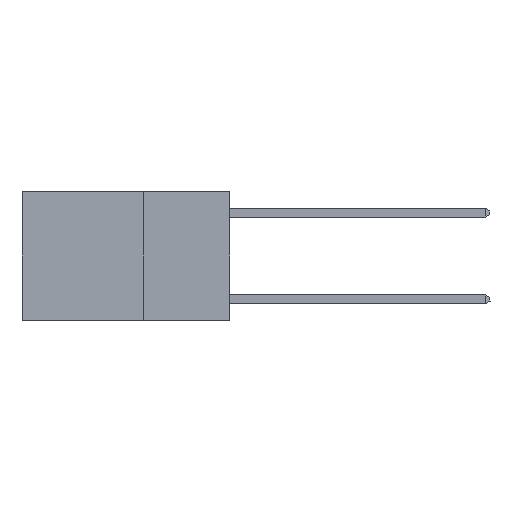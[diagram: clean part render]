
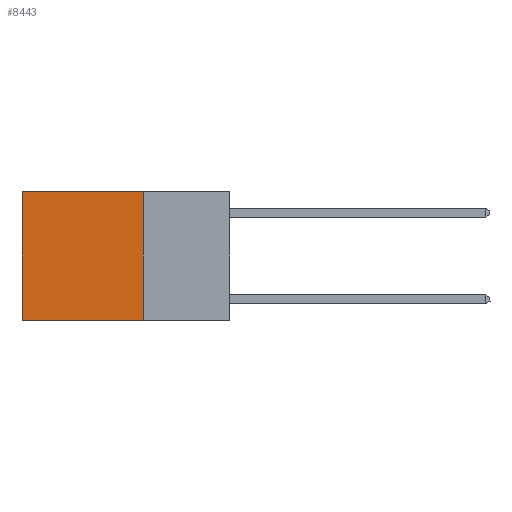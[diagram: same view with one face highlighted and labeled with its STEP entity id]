
A CAD part, left-side view. The second image highlights one B-rep face of the part: STEP entity #8443.
In plain terms, the highlighted planar face has unit normal (-1, 0, 0).
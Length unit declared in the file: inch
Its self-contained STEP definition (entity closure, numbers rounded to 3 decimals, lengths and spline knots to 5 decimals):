
#1500 = DIRECTION ( 'NONE',  ( 0., 1., 0. ) ) ;
#2161 = VECTOR ( 'NONE', #10301, 39.37008 ) ;
#2451 = EDGE_CURVE ( 'NONE', #3620, #8797, #5999, .T. ) ;
#2738 = DIRECTION ( 'NONE',  ( 0., 1., 0. ) ) ;
#3220 = ORIENTED_EDGE ( 'NONE', *, *, #14778, .T. ) ;
#3357 = CARTESIAN_POINT ( 'NONE',  ( 0.2625, 0.25, -0.37 ) ) ;
#3620 = VERTEX_POINT ( 'NONE', #12594 ) ;
#3892 = EDGE_CURVE ( 'NONE', #8797, #12359, #15888, .T. ) ;
#3906 = FACE_OUTER_BOUND ( 'NONE', #12602, .T. ) ;
#4380 = CARTESIAN_POINT ( 'NONE',  ( 0.2625, 0.6, -0.37 ) ) ;
#5059 = ORIENTED_EDGE ( 'NONE', *, *, #3892, .F. ) ;
#5229 = CARTESIAN_POINT ( 'NONE',  ( 0.2625, 0.25, 0. ) ) ;
#5540 = DIRECTION ( 'NONE',  ( 0., 0., -1. ) ) ;
#5999 = LINE ( 'NONE', #5229, #2161 ) ;
#6044 = EDGE_CURVE ( 'NONE', #3620, #12465, #14558, .T. ) ;
#6697 = VECTOR ( 'NONE', #1500, 39.37008 ) ;
#8006 = DIRECTION ( 'NONE',  ( 0., 0., -1. ) ) ;
#8443 = ADVANCED_FACE ( 'NONE', ( #3906 ), #16198, .F. ) ;
#8797 = VERTEX_POINT ( 'NONE', #10371 ) ;
#8907 = LINE ( 'NONE', #12618, #16201 ) ;
#10131 = CARTESIAN_POINT ( 'NONE',  ( 0.2625, 0.25, 0. ) ) ;
#10137 = ORIENTED_EDGE ( 'NONE', *, *, #6044, .T. ) ;
#10271 = CARTESIAN_POINT ( 'NONE',  ( 0.2625, 0.6, 0. ) ) ;
#10301 = DIRECTION ( 'NONE',  ( 0., 0., -1. ) ) ;
#10371 = CARTESIAN_POINT ( 'NONE',  ( 0.2625, 0.25, -0.37 ) ) ;
#11744 = AXIS2_PLACEMENT_3D ( 'NONE', #12188, #16251, #8006 ) ;
#12050 = ORIENTED_EDGE ( 'NONE', *, *, #2451, .F. ) ;
#12188 = CARTESIAN_POINT ( 'NONE',  ( 0.2625, 0.25, 0. ) ) ;
#12301 = VECTOR ( 'NONE', #2738, 39.37008 ) ;
#12359 = VERTEX_POINT ( 'NONE', #4380 ) ;
#12465 = VERTEX_POINT ( 'NONE', #10271 ) ;
#12594 = CARTESIAN_POINT ( 'NONE',  ( 0.2625, 0.25, 0. ) ) ;
#12602 = EDGE_LOOP ( 'NONE', ( #3220, #5059, #12050, #10137 ) ) ;
#12618 = CARTESIAN_POINT ( 'NONE',  ( 0.2625, 0.6, 0. ) ) ;
#14558 = LINE ( 'NONE', #10131, #6697 ) ;
#14778 = EDGE_CURVE ( 'NONE', #12465, #12359, #8907, .T. ) ;
#15888 = LINE ( 'NONE', #3357, #12301 ) ;
#16198 = PLANE ( 'NONE',  #11744 ) ;
#16201 = VECTOR ( 'NONE', #5540, 39.37008 ) ;
#16251 = DIRECTION ( 'NONE',  ( 1., 0., 0. ) ) ;
